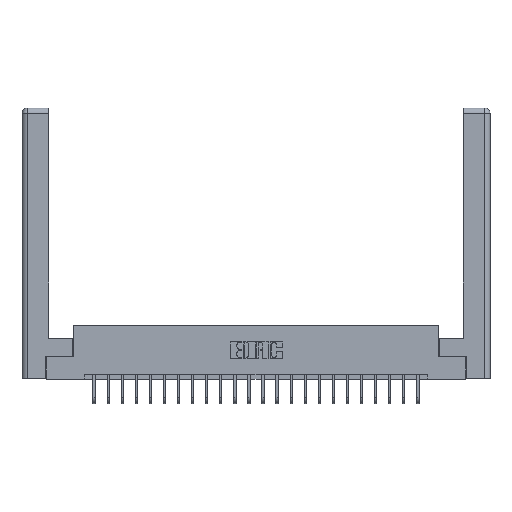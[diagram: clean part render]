
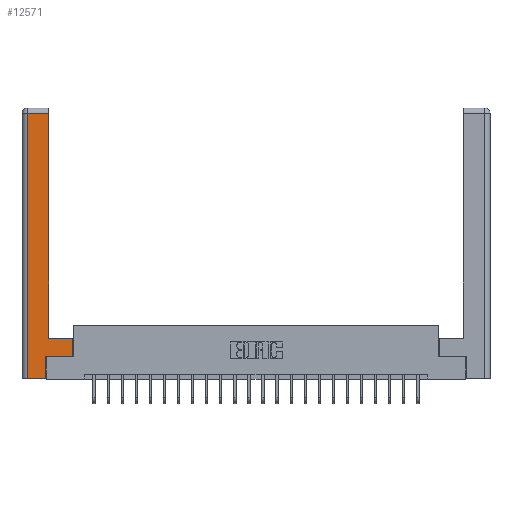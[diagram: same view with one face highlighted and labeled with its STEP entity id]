
A CAD part, top view. The second image highlights one B-rep face of the part: STEP entity #12571.
In plain terms, the highlighted planar face has unit normal (0, 0, 1).
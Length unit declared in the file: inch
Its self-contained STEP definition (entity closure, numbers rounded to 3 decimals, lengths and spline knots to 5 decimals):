
#138 = ORIENTED_EDGE ( 'NONE', *, *, #22865, .T. ) ;
#500 = CARTESIAN_POINT ( 'NONE',  ( 0.565, 0.245, 0. ) ) ;
#527 = DIRECTION ( 'NONE',  ( 0., 1., 0. ) ) ;
#1094 = EDGE_CURVE ( 'NONE', #6237, #14664, #10752, .T. ) ;
#1118 = VECTOR ( 'NONE', #17808, 39.37008 ) ;
#1173 = VECTOR ( 'NONE', #19917, 39.37008 ) ;
#1668 = CARTESIAN_POINT ( 'NONE',  ( 0.265, 0., 0. ) ) ;
#1901 = CARTESIAN_POINT ( 'NONE',  ( 0., 0., 0. ) ) ;
#1979 = DIRECTION ( 'NONE',  ( 0., 0., -1. ) ) ;
#2149 = DIRECTION ( 'NONE',  ( 1., 0., 0. ) ) ;
#2299 = LINE ( 'NONE', #13233, #10930 ) ;
#2320 = VERTEX_POINT ( 'NONE', #18704 ) ;
#2351 = ORIENTED_EDGE ( 'NONE', *, *, #22479, .T. ) ;
#2614 = DIRECTION ( 'NONE',  ( 0., -1., 0. ) ) ;
#3554 = ORIENTED_EDGE ( 'NONE', *, *, #3724, .T. ) ;
#3699 = CARTESIAN_POINT ( 'NONE',  ( 0.265, 0., 0. ) ) ;
#3724 = EDGE_CURVE ( 'NONE', #14664, #5776, #2299, .T. ) ;
#3841 = DIRECTION ( 'NONE',  ( 1., 0., 0. ) ) ;
#3957 = CARTESIAN_POINT ( 'NONE',  ( 0.295, 0.45, 0. ) ) ;
#4263 = CARTESIAN_POINT ( 'NONE',  ( 0.265, 0.245, 0. ) ) ;
#4915 = DIRECTION ( 'NONE',  ( -1., 0., 0. ) ) ;
#5776 = VERTEX_POINT ( 'NONE', #6003 ) ;
#5968 = DIRECTION ( 'NONE',  ( 0., 1., 0. ) ) ;
#6003 = CARTESIAN_POINT ( 'NONE',  ( 0.0615, 0., 0. ) ) ;
#6237 = VERTEX_POINT ( 'NONE', #8674 ) ;
#6572 = VECTOR ( 'NONE', #4915, 39.37008 ) ;
#6857 = ORIENTED_EDGE ( 'NONE', *, *, #21057, .T. ) ;
#7347 = LINE ( 'NONE', #17913, #17867 ) ;
#7597 = ORIENTED_EDGE ( 'NONE', *, *, #1094, .T. ) ;
#8414 = LINE ( 'NONE', #4263, #17544 ) ;
#8674 = CARTESIAN_POINT ( 'NONE',  ( 0.295, 2.94, 0. ) ) ;
#9110 = DIRECTION ( 'NONE',  ( -1., 0., 0. ) ) ;
#9357 = FACE_OUTER_BOUND ( 'NONE', #13595, .T. ) ;
#10209 = EDGE_CURVE ( 'NONE', #19423, #6237, #14171, .T. ) ;
#10732 = AXIS2_PLACEMENT_3D ( 'NONE', #1901, #1979, #9110 ) ;
#10752 = LINE ( 'NONE', #17234, #6572 ) ;
#10930 = VECTOR ( 'NONE', #2614, 39.37008 ) ;
#11764 = CARTESIAN_POINT ( 'NONE',  ( 0.0615, 2.94, 0. ) ) ;
#12121 = EDGE_CURVE ( 'NONE', #5776, #14925, #18457, .T. ) ;
#12436 = CARTESIAN_POINT ( 'NONE',  ( 0.295, 3., 0. ) ) ;
#12571 = ADVANCED_FACE ( 'NONE', ( #9357 ), #19437, .F. ) ;
#13082 = VERTEX_POINT ( 'NONE', #17982 ) ;
#13233 = CARTESIAN_POINT ( 'NONE',  ( 0.0615, 0., 0. ) ) ;
#13595 = EDGE_LOOP ( 'NONE', ( #16833, #7597, #3554, #22118, #138, #6857, #15538, #2351 ) ) ;
#14171 = LINE ( 'NONE', #12436, #1118 ) ;
#14664 = VERTEX_POINT ( 'NONE', #11764 ) ;
#14751 = LINE ( 'NONE', #18153, #1173 ) ;
#14925 = VERTEX_POINT ( 'NONE', #1668 ) ;
#15538 = ORIENTED_EDGE ( 'NONE', *, *, #18977, .T. ) ;
#16833 = ORIENTED_EDGE ( 'NONE', *, *, #10209, .T. ) ;
#17234 = CARTESIAN_POINT ( 'NONE',  ( 0.0615, 2.94, 0. ) ) ;
#17544 = VECTOR ( 'NONE', #527, 39.37008 ) ;
#17644 = VECTOR ( 'NONE', #2149, 39.37008 ) ;
#17808 = DIRECTION ( 'NONE',  ( 0., 1., 0. ) ) ;
#17867 = VECTOR ( 'NONE', #5968, 39.37008 ) ;
#17913 = CARTESIAN_POINT ( 'NONE',  ( 0.565, 0.45, 0. ) ) ;
#17982 = CARTESIAN_POINT ( 'NONE',  ( 0.265, 0.245, 0. ) ) ;
#18153 = CARTESIAN_POINT ( 'NONE',  ( 0.295, 0.45, 0. ) ) ;
#18288 = CARTESIAN_POINT ( 'NONE',  ( 0.565, 0.45, 0. ) ) ;
#18457 = LINE ( 'NONE', #3699, #17644 ) ;
#18704 = CARTESIAN_POINT ( 'NONE',  ( 0.565, 0.245, 0. ) ) ;
#18977 = EDGE_CURVE ( 'NONE', #2320, #20697, #7347, .T. ) ;
#19423 = VERTEX_POINT ( 'NONE', #3957 ) ;
#19437 = PLANE ( 'NONE',  #10732 ) ;
#19917 = DIRECTION ( 'NONE',  ( -1., 0., 0. ) ) ;
#20697 = VERTEX_POINT ( 'NONE', #18288 ) ;
#21057 = EDGE_CURVE ( 'NONE', #13082, #2320, #21962, .T. ) ;
#21407 = VECTOR ( 'NONE', #3841, 39.37008 ) ;
#21962 = LINE ( 'NONE', #500, #21407 ) ;
#22118 = ORIENTED_EDGE ( 'NONE', *, *, #12121, .T. ) ;
#22479 = EDGE_CURVE ( 'NONE', #20697, #19423, #14751, .T. ) ;
#22865 = EDGE_CURVE ( 'NONE', #14925, #13082, #8414, .T. ) ;
